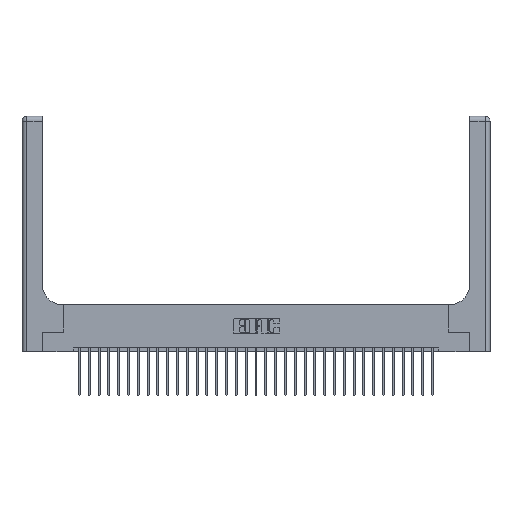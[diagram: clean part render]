
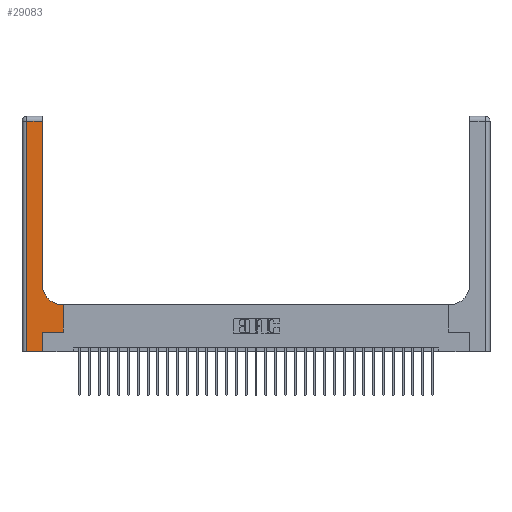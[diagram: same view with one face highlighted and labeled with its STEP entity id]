
A CAD part, top view. The second image highlights one B-rep face of the part: STEP entity #29083.
In plain terms, the highlighted planar face has unit normal (0, 0, 1).
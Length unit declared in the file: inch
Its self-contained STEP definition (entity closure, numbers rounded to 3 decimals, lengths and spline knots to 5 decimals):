
#224 = EDGE_LOOP ( 'NONE', ( #21014, #19997, #1251, #8577, #20609, #16790, #14288, #9118, #11051 ) ) ;
#545 = EDGE_CURVE ( 'NONE', #10506, #16968, #19303, .T. ) ;
#1023 = CARTESIAN_POINT ( 'NONE',  ( 0., 3., 0.37 ) ) ;
#1083 = DIRECTION ( 'NONE',  ( -1., 0., 0. ) ) ;
#1251 = ORIENTED_EDGE ( 'NONE', *, *, #19640, .T. ) ;
#2483 = EDGE_CURVE ( 'NONE', #8690, #2619, #28085, .T. ) ;
#2619 = VERTEX_POINT ( 'NONE', #26807 ) ;
#3111 = LINE ( 'NONE', #5899, #26882 ) ;
#3353 = FACE_OUTER_BOUND ( 'NONE', #224, .T. ) ;
#4167 = DIRECTION ( 'NONE',  ( 0., 1., 0. ) ) ;
#4285 = VERTEX_POINT ( 'NONE', #24988 ) ;
#4614 = EDGE_CURVE ( 'NONE', #8769, #26742, #3111, .T. ) ;
#4891 = VECTOR ( 'NONE', #5423, 39.37008 ) ;
#5423 = DIRECTION ( 'NONE',  ( 0., -1., 0. ) ) ;
#5718 = LINE ( 'NONE', #20544, #10169 ) ;
#5899 = CARTESIAN_POINT ( 'NONE',  ( 0., 2.94, 0.37 ) ) ;
#6895 = EDGE_CURVE ( 'NONE', #12842, #8769, #23586, .T. ) ;
#6996 = LINE ( 'NONE', #9728, #7321 ) ;
#7321 = VECTOR ( 'NONE', #7454, 39.37008 ) ;
#7454 = DIRECTION ( 'NONE',  ( 1., 0., 0. ) ) ;
#7732 = LINE ( 'NONE', #26419, #4891 ) ;
#8577 = ORIENTED_EDGE ( 'NONE', *, *, #22959, .T. ) ;
#8690 = VERTEX_POINT ( 'NONE', #8874 ) ;
#8769 = VERTEX_POINT ( 'NONE', #16466 ) ;
#8874 = CARTESIAN_POINT ( 'NONE',  ( 0.528, 0.6, 0.37 ) ) ;
#9118 = ORIENTED_EDGE ( 'NONE', *, *, #2483, .T. ) ;
#9728 = CARTESIAN_POINT ( 'NONE',  ( 0., 0., 0.37 ) ) ;
#10169 = VECTOR ( 'NONE', #27182, 39.37008 ) ;
#10506 = VERTEX_POINT ( 'NONE', #11623 ) ;
#10984 = EDGE_CURVE ( 'NONE', #4285, #10506, #5718, .T. ) ;
#11051 = ORIENTED_EDGE ( 'NONE', *, *, #25475, .T. ) ;
#11623 = CARTESIAN_POINT ( 'NONE',  ( 0.265, 0.25, 0.37 ) ) ;
#12202 = CARTESIAN_POINT ( 'NONE',  ( 0.265, 0.25, 0.37 ) ) ;
#12842 = VERTEX_POINT ( 'NONE', #20655 ) ;
#14288 = ORIENTED_EDGE ( 'NONE', *, *, #26925, .T. ) ;
#14444 = VERTEX_POINT ( 'NONE', #19427 ) ;
#14686 = CARTESIAN_POINT ( 'NONE',  ( 0.06, 2.94, 0.37 ) ) ;
#14816 = VECTOR ( 'NONE', #4167, 39.37008 ) ;
#15736 = AXIS2_PLACEMENT_3D ( 'NONE', #27748, #29575, #30026 ) ;
#15930 = LINE ( 'NONE', #25322, #14816 ) ;
#16466 = CARTESIAN_POINT ( 'NONE',  ( 0.26, 2.94, 0.37 ) ) ;
#16749 = CIRCLE ( 'NONE', #15736, 0.25 ) ;
#16790 = ORIENTED_EDGE ( 'NONE', *, *, #545, .T. ) ;
#16968 = VERTEX_POINT ( 'NONE', #20392 ) ;
#18808 = DIRECTION ( 'NONE',  ( 0., 1., 0. ) ) ;
#19303 = LINE ( 'NONE', #12202, #28918 ) ;
#19427 = CARTESIAN_POINT ( 'NONE',  ( 0.06, 0., 0.37 ) ) ;
#19640 = EDGE_CURVE ( 'NONE', #26742, #14444, #7732, .T. ) ;
#19997 = ORIENTED_EDGE ( 'NONE', *, *, #4614, .T. ) ;
#20392 = CARTESIAN_POINT ( 'NONE',  ( 0.528, 0.25, 0.37 ) ) ;
#20544 = CARTESIAN_POINT ( 'NONE',  ( 0.265, 0., 0.37 ) ) ;
#20609 = ORIENTED_EDGE ( 'NONE', *, *, #10984, .T. ) ;
#20655 = CARTESIAN_POINT ( 'NONE',  ( 0.26, 0.85, 0.37 ) ) ;
#20782 = VECTOR ( 'NONE', #18808, 39.37008 ) ;
#21014 = ORIENTED_EDGE ( 'NONE', *, *, #6895, .T. ) ;
#21620 = DIRECTION ( 'NONE',  ( 1., 0., 0. ) ) ;
#22743 = AXIS2_PLACEMENT_3D ( 'NONE', #1023, #24823, #29434 ) ;
#22959 = EDGE_CURVE ( 'NONE', #14444, #4285, #6996, .T. ) ;
#23586 = LINE ( 'NONE', #26353, #20782 ) ;
#24658 = VECTOR ( 'NONE', #25769, 39.37008 ) ;
#24823 = DIRECTION ( 'NONE',  ( 0., 0., -1. ) ) ;
#24988 = CARTESIAN_POINT ( 'NONE',  ( 0.265, 0., 0.37 ) ) ;
#25322 = CARTESIAN_POINT ( 'NONE',  ( 0.528, 0.25, 0.37 ) ) ;
#25475 = EDGE_CURVE ( 'NONE', #2619, #12842, #16749, .T. ) ;
#25769 = DIRECTION ( 'NONE',  ( -1., 0., 0. ) ) ;
#26353 = CARTESIAN_POINT ( 'NONE',  ( 0.26, 3., 0.37 ) ) ;
#26419 = CARTESIAN_POINT ( 'NONE',  ( 0.06, 3., 0.37 ) ) ;
#26742 = VERTEX_POINT ( 'NONE', #14686 ) ;
#26807 = CARTESIAN_POINT ( 'NONE',  ( 0.51, 0.6, 0.37 ) ) ;
#26882 = VECTOR ( 'NONE', #1083, 39.37008 ) ;
#26925 = EDGE_CURVE ( 'NONE', #16968, #8690, #15930, .T. ) ;
#26989 = PLANE ( 'NONE',  #22743 ) ;
#27182 = DIRECTION ( 'NONE',  ( 0., 1., 0. ) ) ;
#27748 = CARTESIAN_POINT ( 'NONE',  ( 0.51, 0.85, 0.37 ) ) ;
#28085 = LINE ( 'NONE', #28238, #24658 ) ;
#28238 = CARTESIAN_POINT ( 'NONE',  ( 0.26, 0.6, 0.37 ) ) ;
#28918 = VECTOR ( 'NONE', #21620, 39.37008 ) ;
#29083 = ADVANCED_FACE ( 'NONE', ( #3353 ), #26989, .F. ) ;
#29434 = DIRECTION ( 'NONE',  ( -1., 0., 0. ) ) ;
#29575 = DIRECTION ( 'NONE',  ( 0., 0., -1. ) ) ;
#30026 = DIRECTION ( 'NONE',  ( 1., 0., 0. ) ) ;
